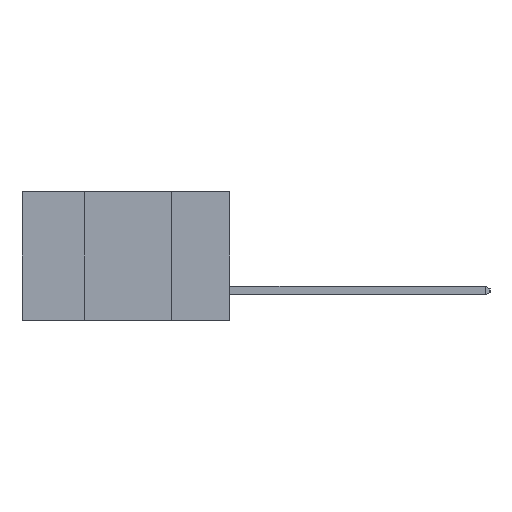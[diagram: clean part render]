
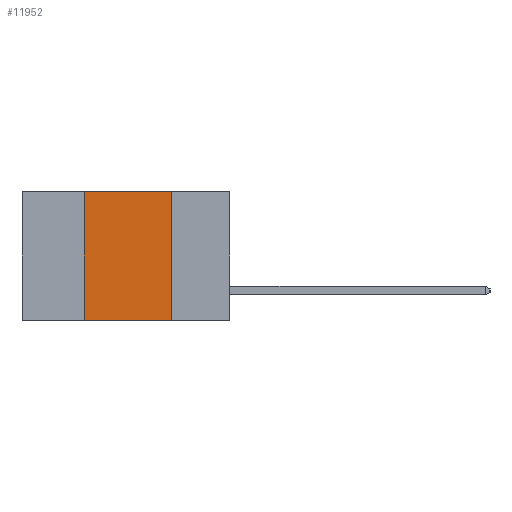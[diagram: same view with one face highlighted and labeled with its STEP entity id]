
A CAD part, left-side view. The second image highlights one B-rep face of the part: STEP entity #11952.
In plain terms, the highlighted planar face has unit normal (-1, 0, 0).
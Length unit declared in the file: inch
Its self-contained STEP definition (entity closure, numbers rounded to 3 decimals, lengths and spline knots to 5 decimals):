
#12 = EDGE_CURVE ( 'NONE', #2882, #5592, #11169, .T. ) ;
#209 = CARTESIAN_POINT ( 'NONE',  ( 0., 0.6, -0.37 ) ) ;
#653 = DIRECTION ( 'NONE',  ( 1., 0., 0. ) ) ;
#1850 = VERTEX_POINT ( 'NONE', #16153 ) ;
#2198 = CARTESIAN_POINT ( 'NONE',  ( 0., 0.42, -0.37 ) ) ;
#2237 = ORIENTED_EDGE ( 'NONE', *, *, #18469, .F. ) ;
#2371 = LINE ( 'NONE', #10077, #16978 ) ;
#2882 = VERTEX_POINT ( 'NONE', #18401 ) ;
#3312 = VERTEX_POINT ( 'NONE', #12555 ) ;
#3337 = DIRECTION ( 'NONE',  ( 0., -1., 0. ) ) ;
#5592 = VERTEX_POINT ( 'NONE', #12288 ) ;
#6617 = VECTOR ( 'NONE', #11120, 39.37008 ) ;
#6743 = EDGE_LOOP ( 'NONE', ( #10514, #8230, #2237, #8532 ) ) ;
#7111 = EDGE_CURVE ( 'NONE', #1850, #3312, #15485, .T. ) ;
#8230 = ORIENTED_EDGE ( 'NONE', *, *, #7111, .F. ) ;
#8487 = EDGE_CURVE ( 'NONE', #3312, #5592, #2371, .T. ) ;
#8532 = ORIENTED_EDGE ( 'NONE', *, *, #12, .T. ) ;
#9274 = FACE_OUTER_BOUND ( 'NONE', #6743, .T. ) ;
#9661 = CARTESIAN_POINT ( 'NONE',  ( 0., 0.6, 0. ) ) ;
#9857 = DIRECTION ( 'NONE',  ( 0., 0., -1. ) ) ;
#10077 = CARTESIAN_POINT ( 'NONE',  ( 0., 0.17, -0.37 ) ) ;
#10514 = ORIENTED_EDGE ( 'NONE', *, *, #8487, .F. ) ;
#10742 = DIRECTION ( 'NONE',  ( 0., -1., 0. ) ) ;
#11120 = DIRECTION ( 'NONE',  ( 0., 0., 1. ) ) ;
#11136 = DIRECTION ( 'NONE',  ( 0., 0., -1. ) ) ;
#11169 = LINE ( 'NONE', #209, #18630 ) ;
#11740 = VECTOR ( 'NONE', #10742, 39.37008 ) ;
#11952 = ADVANCED_FACE ( 'NONE', ( #9274 ), #13934, .F. ) ;
#12288 = CARTESIAN_POINT ( 'NONE',  ( 0., 0.17, -0.37 ) ) ;
#12555 = CARTESIAN_POINT ( 'NONE',  ( 0., 0.17, 0. ) ) ;
#12674 = AXIS2_PLACEMENT_3D ( 'NONE', #9661, #653, #11136 ) ;
#13934 = PLANE ( 'NONE',  #12674 ) ;
#15262 = CARTESIAN_POINT ( 'NONE',  ( 0., 0.6, 0. ) ) ;
#15485 = LINE ( 'NONE', #15262, #11740 ) ;
#16153 = CARTESIAN_POINT ( 'NONE',  ( 0., 0.42, 0. ) ) ;
#16978 = VECTOR ( 'NONE', #9857, 39.37008 ) ;
#17655 = LINE ( 'NONE', #2198, #6617 ) ;
#18401 = CARTESIAN_POINT ( 'NONE',  ( 0., 0.42, -0.37 ) ) ;
#18469 = EDGE_CURVE ( 'NONE', #2882, #1850, #17655, .T. ) ;
#18630 = VECTOR ( 'NONE', #3337, 39.37008 ) ;
